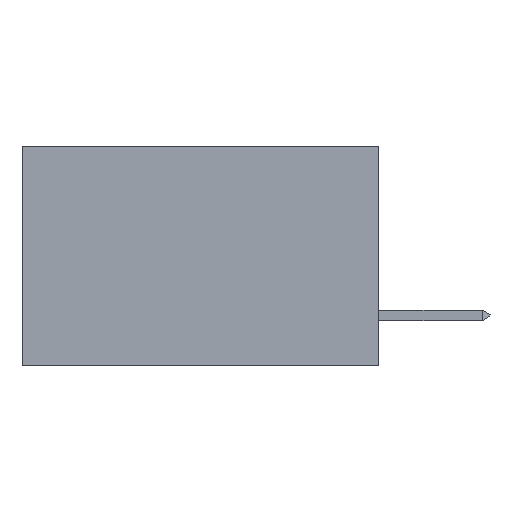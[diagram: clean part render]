
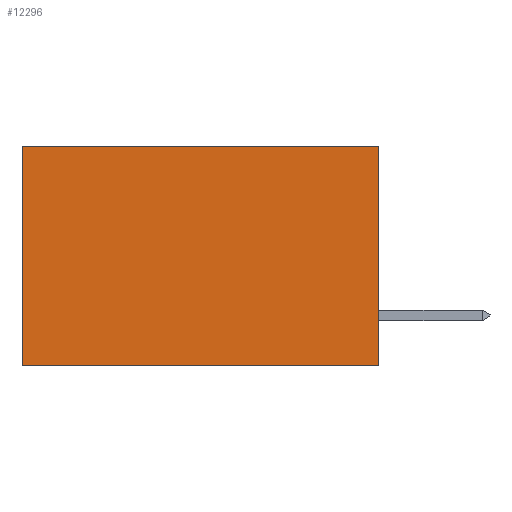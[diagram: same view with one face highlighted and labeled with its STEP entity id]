
A CAD part, left-side view. The second image highlights one B-rep face of the part: STEP entity #12296.
In plain terms, the highlighted planar face has unit normal (-1, 0, 0).
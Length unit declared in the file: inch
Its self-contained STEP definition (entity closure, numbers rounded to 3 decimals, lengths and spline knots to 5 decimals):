
#135 = VECTOR ( 'NONE', #3077, 39.37008 ) ;
#362 = CARTESIAN_POINT ( 'NONE',  ( 0.298, 0.6, -0.37 ) ) ;
#860 = AXIS2_PLACEMENT_3D ( 'NONE', #12391, #12471, #8199 ) ;
#990 = DIRECTION ( 'NONE',  ( 0., 1., 0. ) ) ;
#1290 = VECTOR ( 'NONE', #1634, 39.37008 ) ;
#1634 = DIRECTION ( 'NONE',  ( 0., 1., 0. ) ) ;
#1898 = CARTESIAN_POINT ( 'NONE',  ( 0.298, 0., -0.37 ) ) ;
#1917 = VECTOR ( 'NONE', #6519, 39.37008 ) ;
#2367 = CARTESIAN_POINT ( 'NONE',  ( 0.298, 0., 0. ) ) ;
#2624 = VERTEX_POINT ( 'NONE', #362 ) ;
#3077 = DIRECTION ( 'NONE',  ( 0., 0., -1. ) ) ;
#3694 = CARTESIAN_POINT ( 'NONE',  ( 0.298, 0.6, 0. ) ) ;
#3919 = CARTESIAN_POINT ( 'NONE',  ( 0.298, 0., 0. ) ) ;
#3997 = EDGE_LOOP ( 'NONE', ( #5698, #5638, #7826, #8370 ) ) ;
#4133 = VERTEX_POINT ( 'NONE', #3694 ) ;
#4174 = EDGE_CURVE ( 'NONE', #11164, #4746, #5853, .T. ) ;
#4700 = CARTESIAN_POINT ( 'NONE',  ( 0.298, 0., 0. ) ) ;
#4746 = VERTEX_POINT ( 'NONE', #1898 ) ;
#5060 = CARTESIAN_POINT ( 'NONE',  ( 0.298, 0.6, 0. ) ) ;
#5488 = CARTESIAN_POINT ( 'NONE',  ( 0.298, 0., -0.37 ) ) ;
#5638 = ORIENTED_EDGE ( 'NONE', *, *, #11722, .F. ) ;
#5698 = ORIENTED_EDGE ( 'NONE', *, *, #10631, .T. ) ;
#5853 = LINE ( 'NONE', #4700, #1917 ) ;
#6170 = FACE_OUTER_BOUND ( 'NONE', #3997, .T. ) ;
#6519 = DIRECTION ( 'NONE',  ( 0., 0., -1. ) ) ;
#7424 = VECTOR ( 'NONE', #990, 39.37008 ) ;
#7698 = EDGE_CURVE ( 'NONE', #11164, #4133, #9238, .T. ) ;
#7826 = ORIENTED_EDGE ( 'NONE', *, *, #4174, .F. ) ;
#8199 = DIRECTION ( 'NONE',  ( 0., 0., -1. ) ) ;
#8370 = ORIENTED_EDGE ( 'NONE', *, *, #7698, .T. ) ;
#9238 = LINE ( 'NONE', #3919, #7424 ) ;
#10157 = PLANE ( 'NONE',  #860 ) ;
#10482 = LINE ( 'NONE', #5060, #135 ) ;
#10631 = EDGE_CURVE ( 'NONE', #4133, #2624, #10482, .T. ) ;
#11164 = VERTEX_POINT ( 'NONE', #2367 ) ;
#11722 = EDGE_CURVE ( 'NONE', #4746, #2624, #11818, .T. ) ;
#11818 = LINE ( 'NONE', #5488, #1290 ) ;
#12296 = ADVANCED_FACE ( 'NONE', ( #6170 ), #10157, .F. ) ;
#12391 = CARTESIAN_POINT ( 'NONE',  ( 0.298, 0., 0. ) ) ;
#12471 = DIRECTION ( 'NONE',  ( 1., 0., 0. ) ) ;
